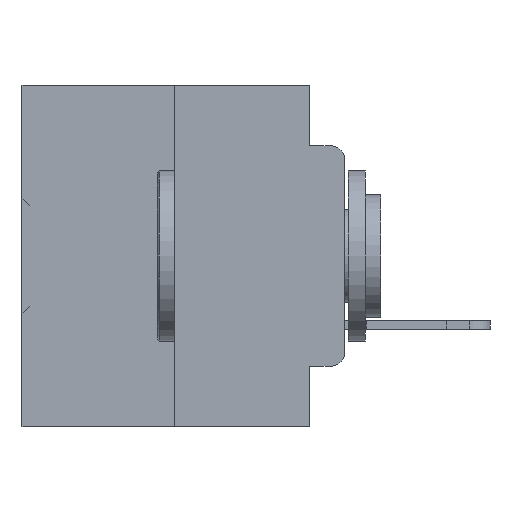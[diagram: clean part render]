
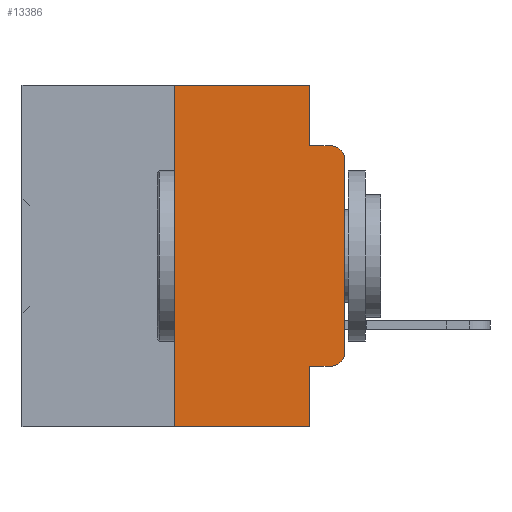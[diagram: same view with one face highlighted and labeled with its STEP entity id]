
A CAD part, left-side view. The second image highlights one B-rep face of the part: STEP entity #13386.
In plain terms, the highlighted planar face has unit normal (-1, 0, 0).
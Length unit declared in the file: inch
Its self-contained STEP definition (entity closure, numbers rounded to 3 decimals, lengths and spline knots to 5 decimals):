
#214 = ORIENTED_EDGE ( 'NONE', *, *, #15550, .T. ) ;
#712 = VECTOR ( 'NONE', #7341, 39.37008 ) ;
#893 = VERTEX_POINT ( 'NONE', #14372 ) ;
#1930 = DIRECTION ( 'NONE',  ( 0., 0., -1. ) ) ;
#1941 = DIRECTION ( 'NONE',  ( 1., 0., 0. ) ) ;
#2186 = PLANE ( 'NONE',  #18064 ) ;
#2305 = CIRCLE ( 'NONE', #4563, 0.02 ) ;
#2658 = CARTESIAN_POINT ( 'NONE',  ( 0., 0.473, 0. ) ) ;
#2721 = VECTOR ( 'NONE', #35945, 39.37008 ) ;
#2761 = LINE ( 'NONE', #37537, #32880 ) ;
#3226 = VERTEX_POINT ( 'NONE', #8593 ) ;
#3559 = VERTEX_POINT ( 'NONE', #26587 ) ;
#3580 = EDGE_CURVE ( 'NONE', #12583, #17037, #18431, .T. ) ;
#4563 = AXIS2_PLACEMENT_3D ( 'NONE', #7496, #7416, #7404 ) ;
#5562 = ORIENTED_EDGE ( 'NONE', *, *, #7140, .F. ) ;
#6572 = FACE_OUTER_BOUND ( 'NONE', #7391, .T. ) ;
#7140 = EDGE_CURVE ( 'NONE', #16240, #3226, #27677, .T. ) ;
#7341 = DIRECTION ( 'NONE',  ( 0., 0., 1. ) ) ;
#7391 = EDGE_LOOP ( 'NONE', ( #13457, #214, #5562, #18301, #18461, #26111, #19638, #13798, #9720, #33653 ) ) ;
#7404 = DIRECTION ( 'NONE',  ( 0., 0., -1. ) ) ;
#7416 = DIRECTION ( 'NONE',  ( -1., 0., 0. ) ) ;
#7496 = CARTESIAN_POINT ( 'NONE',  ( 0., 0.02, -0.1085 ) ) ;
#8593 = CARTESIAN_POINT ( 'NONE',  ( 0., 0.02, -0.0885 ) ) ;
#9146 = VECTOR ( 'NONE', #27935, 39.37008 ) ;
#9720 = ORIENTED_EDGE ( 'NONE', *, *, #33849, .T. ) ;
#11613 = VECTOR ( 'NONE', #20917, 39.37008 ) ;
#11887 = VECTOR ( 'NONE', #16748, 39.37008 ) ;
#12583 = VERTEX_POINT ( 'NONE', #16095 ) ;
#12934 = VERTEX_POINT ( 'NONE', #27420 ) ;
#13386 = ADVANCED_FACE ( 'NONE', ( #6572 ), #2186, .F. ) ;
#13402 = CARTESIAN_POINT ( 'NONE',  ( 0., 0.02, -0.3915 ) ) ;
#13457 = ORIENTED_EDGE ( 'NONE', *, *, #21474, .T. ) ;
#13798 = ORIENTED_EDGE ( 'NONE', *, *, #3580, .F. ) ;
#13968 = CIRCLE ( 'NONE', #33016, 0.02 ) ;
#14372 = CARTESIAN_POINT ( 'NONE',  ( 0., 0.02, -0.4115 ) ) ;
#15550 = EDGE_CURVE ( 'NONE', #24964, #3226, #2305, .T. ) ;
#15644 = VECTOR ( 'NONE', #25580, 39.37008 ) ;
#15980 = VECTOR ( 'NONE', #32860, 39.37008 ) ;
#16088 = CARTESIAN_POINT ( 'NONE',  ( 0., 0.051, -0.0885 ) ) ;
#16095 = CARTESIAN_POINT ( 'NONE',  ( 0., 0.051, -0.4115 ) ) ;
#16153 = EDGE_CURVE ( 'NONE', #3559, #12934, #2761, .T. ) ;
#16240 = VERTEX_POINT ( 'NONE', #33590 ) ;
#16491 = DIRECTION ( 'NONE',  ( 0., 0., -1. ) ) ;
#16748 = DIRECTION ( 'NONE',  ( 0., -1., 0. ) ) ;
#17037 = VERTEX_POINT ( 'NONE', #34232 ) ;
#17637 = LINE ( 'NONE', #31256, #712 ) ;
#18064 = AXIS2_PLACEMENT_3D ( 'NONE', #2658, #1941, #1930 ) ;
#18301 = ORIENTED_EDGE ( 'NONE', *, *, #26145, .F. ) ;
#18431 = LINE ( 'NONE', #25706, #15644 ) ;
#18461 = ORIENTED_EDGE ( 'NONE', *, *, #16153, .F. ) ;
#19132 = CARTESIAN_POINT ( 'NONE',  ( 0., 0.051, 0. ) ) ;
#19638 = ORIENTED_EDGE ( 'NONE', *, *, #25283, .T. ) ;
#20241 = EDGE_CURVE ( 'NONE', #33597, #3559, #17637, .T. ) ;
#20557 = LINE ( 'NONE', #35093, #11613 ) ;
#20917 = DIRECTION ( 'NONE',  ( 0., -1., 0. ) ) ;
#21474 = EDGE_CURVE ( 'NONE', #36455, #24964, #27165, .T. ) ;
#22759 = CARTESIAN_POINT ( 'NONE',  ( 0., 0., -0.3915 ) ) ;
#23174 = CARTESIAN_POINT ( 'NONE',  ( 0., 0., -0.1085 ) ) ;
#24964 = VERTEX_POINT ( 'NONE', #23174 ) ;
#25283 = EDGE_CURVE ( 'NONE', #33597, #17037, #31376, .T. ) ;
#25580 = DIRECTION ( 'NONE',  ( 0., 0., -1. ) ) ;
#25706 = CARTESIAN_POINT ( 'NONE',  ( 0., 0.051, 0. ) ) ;
#26085 = LINE ( 'NONE', #19132, #9146 ) ;
#26111 = ORIENTED_EDGE ( 'NONE', *, *, #20241, .F. ) ;
#26145 = EDGE_CURVE ( 'NONE', #12934, #16240, #26085, .T. ) ;
#26587 = CARTESIAN_POINT ( 'NONE',  ( 0., 0.25, 0. ) ) ;
#27067 = EDGE_CURVE ( 'NONE', #893, #36455, #13968, .T. ) ;
#27165 = LINE ( 'NONE', #33230, #2721 ) ;
#27420 = CARTESIAN_POINT ( 'NONE',  ( 0., 0.051, 0. ) ) ;
#27677 = LINE ( 'NONE', #16088, #11887 ) ;
#27935 = DIRECTION ( 'NONE',  ( 0., 0., -1. ) ) ;
#28826 = CARTESIAN_POINT ( 'NONE',  ( 0., 0.25, -0.5 ) ) ;
#31256 = CARTESIAN_POINT ( 'NONE',  ( 0., 0.25, 0. ) ) ;
#31376 = LINE ( 'NONE', #35596, #15980 ) ;
#32860 = DIRECTION ( 'NONE',  ( 0., -1., 0. ) ) ;
#32880 = VECTOR ( 'NONE', #37543, 39.37008 ) ;
#33016 = AXIS2_PLACEMENT_3D ( 'NONE', #13402, #33738, #16491 ) ;
#33230 = CARTESIAN_POINT ( 'NONE',  ( 0., 0., 0. ) ) ;
#33590 = CARTESIAN_POINT ( 'NONE',  ( 0., 0.051, -0.0885 ) ) ;
#33597 = VERTEX_POINT ( 'NONE', #28826 ) ;
#33653 = ORIENTED_EDGE ( 'NONE', *, *, #27067, .T. ) ;
#33738 = DIRECTION ( 'NONE',  ( -1., 0., 0. ) ) ;
#33849 = EDGE_CURVE ( 'NONE', #12583, #893, #20557, .T. ) ;
#34232 = CARTESIAN_POINT ( 'NONE',  ( 0., 0.051, -0.5 ) ) ;
#35093 = CARTESIAN_POINT ( 'NONE',  ( 0., 0.051, -0.4115 ) ) ;
#35596 = CARTESIAN_POINT ( 'NONE',  ( 0., 0.473, -0.5 ) ) ;
#35945 = DIRECTION ( 'NONE',  ( 0., 0., 1. ) ) ;
#36455 = VERTEX_POINT ( 'NONE', #22759 ) ;
#37537 = CARTESIAN_POINT ( 'NONE',  ( 0., 0.473, 0. ) ) ;
#37543 = DIRECTION ( 'NONE',  ( 0., -1., 0. ) ) ;
